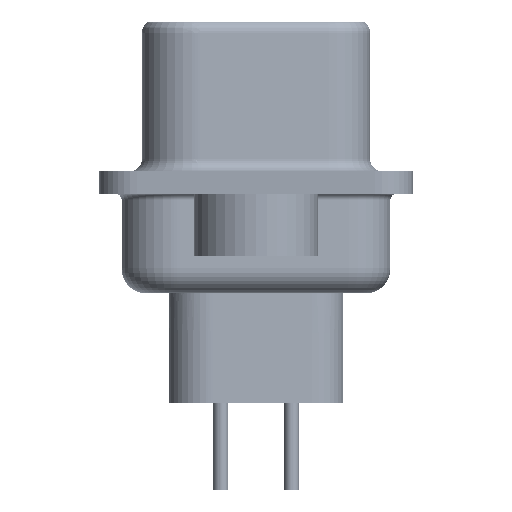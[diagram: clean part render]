
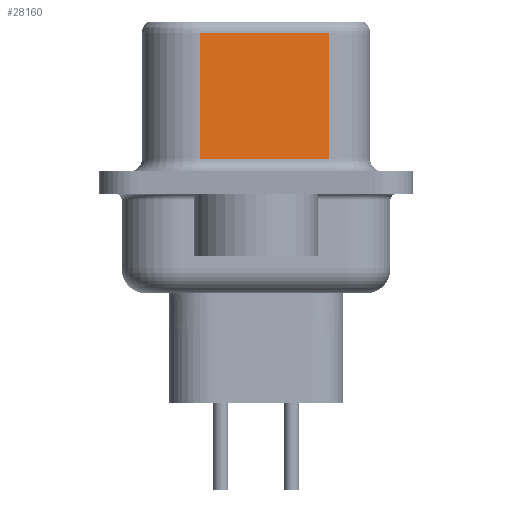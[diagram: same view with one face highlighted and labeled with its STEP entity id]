
A CAD part, left-side view. The second image highlights one B-rep face of the part: STEP entity #28160.
In plain terms, the highlighted planar face has unit normal (-0.985, -0.174, 0).
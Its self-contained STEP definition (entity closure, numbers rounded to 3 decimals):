
#355 = VECTOR ( 'NONE', #19587, 1000. ) ;
#2621 = VERTEX_POINT ( 'NONE', #31990 ) ;
#3645 = CARTESIAN_POINT ( 'NONE',  ( 4.58, -2.927, 6.52 ) ) ;
#4164 = LINE ( 'NONE', #16957, #355 ) ;
#4291 = ORIENTED_EDGE ( 'NONE', *, *, #14723, .T. ) ;
#4853 = VECTOR ( 'NONE', #11963, 1000. ) ;
#5957 = DIRECTION ( 'NONE',  ( 0.985, 0.174, 0. ) ) ;
#8430 = PLANE ( 'NONE',  #10061 ) ;
#9500 = CARTESIAN_POINT ( 'NONE',  ( 4.58, -2.927, 6.02 ) ) ;
#10061 = AXIS2_PLACEMENT_3D ( 'NONE', #28495, #5957, #15962 ) ;
#10772 = CARTESIAN_POINT ( 'NONE',  ( 3.67, 2.233, 6.52 ) ) ;
#11963 = DIRECTION ( 'NONE',  ( -0.174, 0.985, 0. ) ) ;
#13657 = DIRECTION ( 'NONE',  ( 0., 0., -1. ) ) ;
#13828 = VERTEX_POINT ( 'NONE', #20749 ) ;
#14076 = EDGE_CURVE ( 'NONE', #2621, #17161, #15966, .T. ) ;
#14723 = EDGE_CURVE ( 'NONE', #13828, #31752, #22662, .T. ) ;
#15962 = DIRECTION ( 'NONE',  ( -0.174, 0.985, 0. ) ) ;
#15966 = LINE ( 'NONE', #3645, #21218 ) ;
#16157 = CARTESIAN_POINT ( 'NONE',  ( 3.67, 2.233, 0.95 ) ) ;
#16957 = CARTESIAN_POINT ( 'NONE',  ( 4.58, -2.927, 0.95 ) ) ;
#17161 = VERTEX_POINT ( 'NONE', #30109 ) ;
#17385 = DIRECTION ( 'NONE',  ( 0., 0., -1. ) ) ;
#19587 = DIRECTION ( 'NONE',  ( 0.174, -0.985, 0. ) ) ;
#20749 = CARTESIAN_POINT ( 'NONE',  ( 3.67, 2.233, 6.02 ) ) ;
#21218 = VECTOR ( 'NONE', #13657, 1000. ) ;
#22489 = LINE ( 'NONE', #9500, #4853 ) ;
#22662 = LINE ( 'NONE', #10772, #27057 ) ;
#23371 = FACE_OUTER_BOUND ( 'NONE', #29548, .T. ) ;
#24683 = ORIENTED_EDGE ( 'NONE', *, *, #31886, .T. ) ;
#25375 = ORIENTED_EDGE ( 'NONE', *, *, #26256, .T. ) ;
#26256 = EDGE_CURVE ( 'NONE', #2621, #13828, #22489, .T. ) ;
#27057 = VECTOR ( 'NONE', #17385, 1000. ) ;
#28160 = ADVANCED_FACE ( 'NONE', ( #23371 ), #8430, .F. ) ;
#28495 = CARTESIAN_POINT ( 'NONE',  ( 4.58, -2.927, 6.52 ) ) ;
#29548 = EDGE_LOOP ( 'NONE', ( #29900, #25375, #4291, #24683 ) ) ;
#29900 = ORIENTED_EDGE ( 'NONE', *, *, #14076, .F. ) ;
#30109 = CARTESIAN_POINT ( 'NONE',  ( 4.58, -2.927, 0.95 ) ) ;
#31752 = VERTEX_POINT ( 'NONE', #16157 ) ;
#31886 = EDGE_CURVE ( 'NONE', #31752, #17161, #4164, .T. ) ;
#31990 = CARTESIAN_POINT ( 'NONE',  ( 4.58, -2.927, 6.02 ) ) ;
